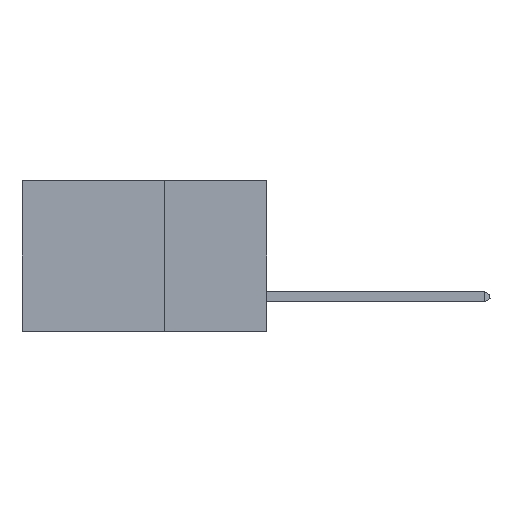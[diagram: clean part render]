
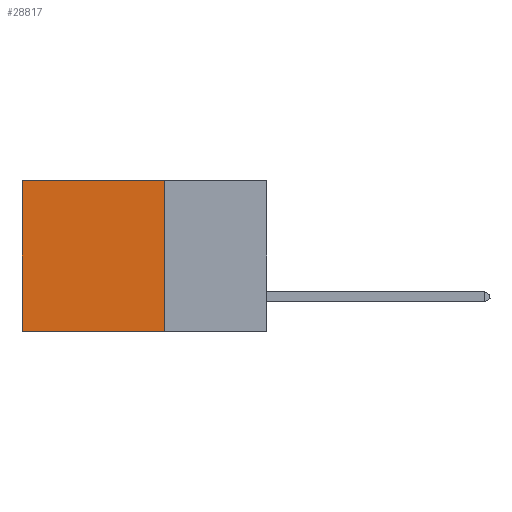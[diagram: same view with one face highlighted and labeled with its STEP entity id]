
A CAD part, left-side view. The second image highlights one B-rep face of the part: STEP entity #28817.
In plain terms, the highlighted planar face has unit normal (-1, 0, 0).
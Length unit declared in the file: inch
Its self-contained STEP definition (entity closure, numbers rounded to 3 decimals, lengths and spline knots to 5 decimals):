
#1269 = AXIS2_PLACEMENT_3D ( 'NONE', #32900, #35573, #23296 ) ;
#3625 = LINE ( 'NONE', #35173, #4580 ) ;
#4106 = FACE_OUTER_BOUND ( 'NONE', #32242, .T. ) ;
#4301 = LINE ( 'NONE', #14601, #17210 ) ;
#4580 = VECTOR ( 'NONE', #13063, 39.37008 ) ;
#6456 = VERTEX_POINT ( 'NONE', #9450 ) ;
#9218 = EDGE_CURVE ( 'NONE', #31795, #20286, #3625, .T. ) ;
#9450 = CARTESIAN_POINT ( 'NONE',  ( 0.2875, 0.25, 0. ) ) ;
#10326 = CARTESIAN_POINT ( 'NONE',  ( 0.2875, 0.6, 0. ) ) ;
#11357 = CARTESIAN_POINT ( 'NONE',  ( 0.2875, 0.6, -0.37 ) ) ;
#12038 = VECTOR ( 'NONE', #39180, 39.37008 ) ;
#13063 = DIRECTION ( 'NONE',  ( 0., 1., 0. ) ) ;
#14601 = CARTESIAN_POINT ( 'NONE',  ( 0.2875, 0.25, 0. ) ) ;
#17210 = VECTOR ( 'NONE', #39241, 39.37008 ) ;
#17340 = CARTESIAN_POINT ( 'NONE',  ( 0.2875, 0.25, -0.37 ) ) ;
#18191 = EDGE_CURVE ( 'NONE', #21190, #20286, #28306, .T. ) ;
#20286 = VERTEX_POINT ( 'NONE', #11357 ) ;
#21061 = ORIENTED_EDGE ( 'NONE', *, *, #18191, .T. ) ;
#21190 = VERTEX_POINT ( 'NONE', #10326 ) ;
#23296 = DIRECTION ( 'NONE',  ( 0., 0., -1. ) ) ;
#24565 = CARTESIAN_POINT ( 'NONE',  ( 0.2875, 0.25, 0. ) ) ;
#26731 = CARTESIAN_POINT ( 'NONE',  ( 0.2875, 0.6, 0. ) ) ;
#28306 = LINE ( 'NONE', #26731, #12038 ) ;
#28658 = ORIENTED_EDGE ( 'NONE', *, *, #32186, .F. ) ;
#28817 = ADVANCED_FACE ( 'NONE', ( #4106 ), #32371, .F. ) ;
#30700 = DIRECTION ( 'NONE',  ( 0., 0., -1. ) ) ;
#31070 = LINE ( 'NONE', #24565, #32014 ) ;
#31795 = VERTEX_POINT ( 'NONE', #17340 ) ;
#32014 = VECTOR ( 'NONE', #30700, 39.37008 ) ;
#32186 = EDGE_CURVE ( 'NONE', #6456, #31795, #31070, .T. ) ;
#32242 = EDGE_LOOP ( 'NONE', ( #21061, #35107, #28658, #34642 ) ) ;
#32371 = PLANE ( 'NONE',  #1269 ) ;
#32659 = EDGE_CURVE ( 'NONE', #6456, #21190, #4301, .T. ) ;
#32900 = CARTESIAN_POINT ( 'NONE',  ( 0.2875, 0.25, 0. ) ) ;
#34642 = ORIENTED_EDGE ( 'NONE', *, *, #32659, .T. ) ;
#35107 = ORIENTED_EDGE ( 'NONE', *, *, #9218, .F. ) ;
#35173 = CARTESIAN_POINT ( 'NONE',  ( 0.2875, 0.25, -0.37 ) ) ;
#35573 = DIRECTION ( 'NONE',  ( 1., 0., 0. ) ) ;
#39180 = DIRECTION ( 'NONE',  ( 0., 0., -1. ) ) ;
#39241 = DIRECTION ( 'NONE',  ( 0., 1., 0. ) ) ;
